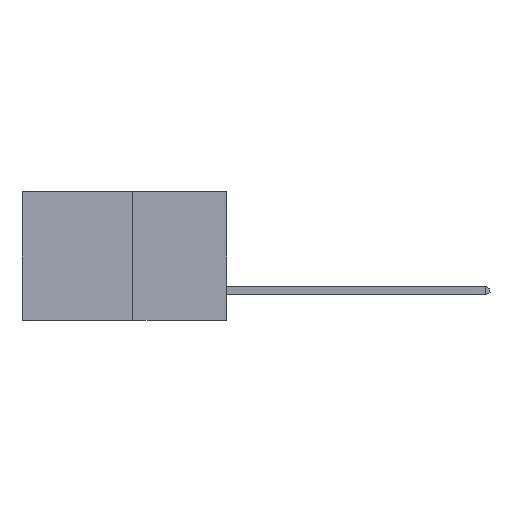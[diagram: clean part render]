
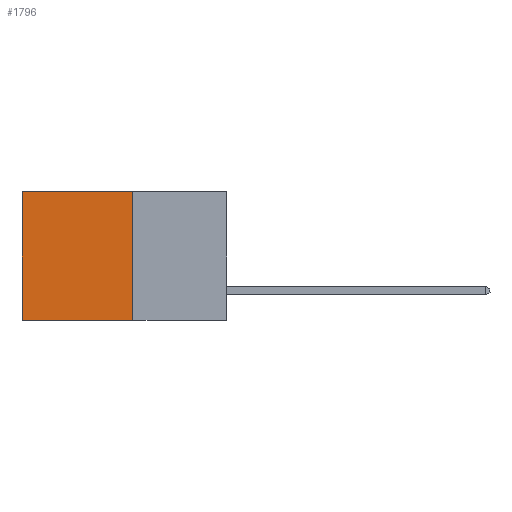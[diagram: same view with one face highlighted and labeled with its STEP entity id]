
A CAD part, left-side view. The second image highlights one B-rep face of the part: STEP entity #1796.
In plain terms, the highlighted planar face has unit normal (-1, 0, 0).
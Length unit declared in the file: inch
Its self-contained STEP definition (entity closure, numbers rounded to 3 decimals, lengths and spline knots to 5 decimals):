
#239 = CARTESIAN_POINT ( 'NONE',  ( 0.277, 0.27, 0. ) ) ;
#265 = ORIENTED_EDGE ( 'NONE', *, *, #7476, .T. ) ;
#276 = ORIENTED_EDGE ( 'NONE', *, *, #1260, .F. ) ;
#564 = LINE ( 'NONE', #6381, #3031 ) ;
#591 = DIRECTION ( 'NONE',  ( 0., 1., 0. ) ) ;
#661 = ORIENTED_EDGE ( 'NONE', *, *, #3988, .F. ) ;
#827 = ORIENTED_EDGE ( 'NONE', *, *, #5649, .T. ) ;
#856 = VERTEX_POINT ( 'NONE', #4181 ) ;
#934 = CARTESIAN_POINT ( 'NONE',  ( 0.277, 0.27, -0.37 ) ) ;
#1260 = EDGE_CURVE ( 'NONE', #3052, #856, #4776, .T. ) ;
#1355 = AXIS2_PLACEMENT_3D ( 'NONE', #934, #3399, #10047 ) ;
#1667 = DIRECTION ( 'NONE',  ( 0., 0., -1. ) ) ;
#1677 = VECTOR ( 'NONE', #591, 39.37008 ) ;
#1796 = ADVANCED_FACE ( 'NONE', ( #4159 ), #8393, .F. ) ;
#2248 = VECTOR ( 'NONE', #1667, 39.37008 ) ;
#2395 = CARTESIAN_POINT ( 'NONE',  ( 0.277, 0.59, -0.37 ) ) ;
#3015 = VERTEX_POINT ( 'NONE', #7711 ) ;
#3031 = VECTOR ( 'NONE', #6344, 39.37008 ) ;
#3052 = VERTEX_POINT ( 'NONE', #8675 ) ;
#3399 = DIRECTION ( 'NONE',  ( 1., 0., 0. ) ) ;
#3988 = EDGE_CURVE ( 'NONE', #856, #4369, #5384, .T. ) ;
#4159 = FACE_OUTER_BOUND ( 'NONE', #6468, .T. ) ;
#4181 = CARTESIAN_POINT ( 'NONE',  ( 0.277, 0.27, -0.37 ) ) ;
#4369 = VERTEX_POINT ( 'NONE', #2395 ) ;
#4776 = LINE ( 'NONE', #9288, #2248 ) ;
#5384 = LINE ( 'NONE', #5684, #9327 ) ;
#5649 = EDGE_CURVE ( 'NONE', #3015, #4369, #564, .T. ) ;
#5684 = CARTESIAN_POINT ( 'NONE',  ( 0.277, 0.27, -0.37 ) ) ;
#5766 = DIRECTION ( 'NONE',  ( 0., 1., 0. ) ) ;
#6169 = LINE ( 'NONE', #239, #1677 ) ;
#6344 = DIRECTION ( 'NONE',  ( 0., 0., -1. ) ) ;
#6381 = CARTESIAN_POINT ( 'NONE',  ( 0.277, 0.59, -0.37 ) ) ;
#6468 = EDGE_LOOP ( 'NONE', ( #827, #661, #276, #265 ) ) ;
#7476 = EDGE_CURVE ( 'NONE', #3052, #3015, #6169, .T. ) ;
#7711 = CARTESIAN_POINT ( 'NONE',  ( 0.277, 0.59, 0. ) ) ;
#8393 = PLANE ( 'NONE',  #1355 ) ;
#8675 = CARTESIAN_POINT ( 'NONE',  ( 0.277, 0.27, 0. ) ) ;
#9288 = CARTESIAN_POINT ( 'NONE',  ( 0.277, 0.27, -0.37 ) ) ;
#9327 = VECTOR ( 'NONE', #5766, 39.37008 ) ;
#10047 = DIRECTION ( 'NONE',  ( 0., 0., -1. ) ) ;
